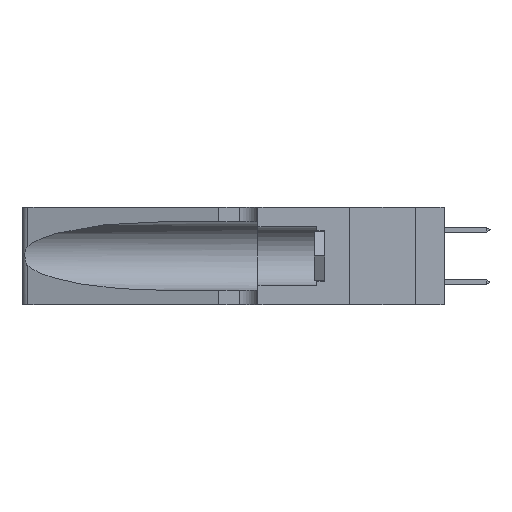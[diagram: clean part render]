
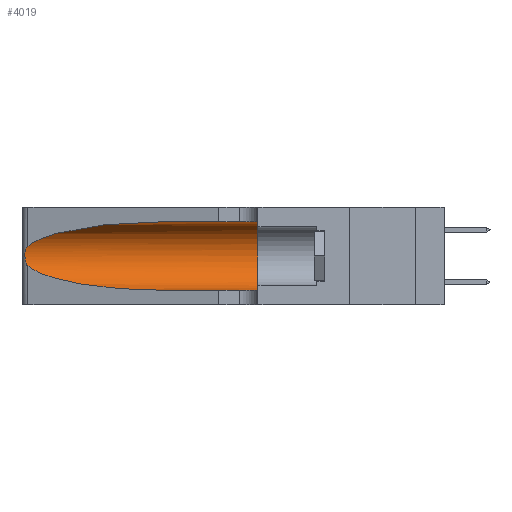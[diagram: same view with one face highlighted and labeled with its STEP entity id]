
A CAD part, left-side view. The second image highlights one B-rep face of the part: STEP entity #4019.
In plain terms, the highlighted cylindrical face has radius 3.308 mm (diameter 6.617 mm), a partial arc.
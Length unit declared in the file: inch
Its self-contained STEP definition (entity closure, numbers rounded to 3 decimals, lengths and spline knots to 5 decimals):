
#219 = CYLINDRICAL_SURFACE ( 'NONE', #3198, 0.13025 ) ;
#246 =( BOUNDED_CURVE ( )  B_SPLINE_CURVE ( 3, ( #7009, #28054, #13171, #34057 ),
 .UNSPECIFIED., .F., .F. ) 
 B_SPLINE_CURVE_WITH_KNOTS ( ( 4, 4 ),
 ( 3.44316, 4.71239 ),
 .UNSPECIFIED. ) 
 CURVE ( )  GEOMETRIC_REPRESENTATION_ITEM ( )  RATIONAL_B_SPLINE_CURVE ( ( 1., 0.87, 0.87, 1. ) ) 
 REPRESENTATION_ITEM ( '' )  );
#276 = CIRCLE ( 'NONE', #25383, 0.13025 ) ;
#822 = EDGE_LOOP ( 'NONE', ( #23058, #15701, #1438, #12077, #12701, #24550 ) ) ;
#1438 = ORIENTED_EDGE ( 'NONE', *, *, #38357, .T. ) ;
#1508 = EDGE_CURVE ( 'NONE', #5871, #12690, #15813, .T. ) ;
#1624 = CARTESIAN_POINT ( 'NONE',  ( 0.25487, 1.22718, 0.14631 ) ) ;
#2170 = CARTESIAN_POINT ( 'NONE',  ( 0.1305, 0.35, 0.31525 ) ) ;
#2357 = CARTESIAN_POINT ( 'NONE',  ( 0.25487, 1.22718, 0.22369 ) ) ;
#2413 = B_SPLINE_CURVE_WITH_KNOTS ( 'NONE', 3,
 ( #38286, #2547, #23443, #5519, #26438, #8510, #29458, #11531, #32445, #14548, #35421, #17577, #38415, #20570 ),
 .UNSPECIFIED., .F., .F.,
 ( 4, 2, 2, 2, 2, 2, 4 ),
 ( 0., 0.00027, 0.00053, 0.00107, 0.0016, 0.00187, 0.00214 ),
 .UNSPECIFIED. ) ;
#2547 = CARTESIAN_POINT ( 'NONE',  ( 0.25555, 1.22994, 0.2215 ) ) ;
#3198 = AXIS2_PLACEMENT_3D ( 'NONE', #16350, #31252, #37197 ) ;
#4019 = ADVANCED_FACE ( 'NONE', ( #16087 ), #219, .F. ) ;
#4147 = VECTOR ( 'NONE', #25179, 39.37008 ) ;
#5519 = CARTESIAN_POINT ( 'NONE',  ( 0.25787, 1.23484, 0.2124 ) ) ;
#5871 = VERTEX_POINT ( 'NONE', #16844 ) ;
#6707 = CARTESIAN_POINT ( 'NONE',  ( 0.1305, 0.35, 0.185 ) ) ;
#7009 = CARTESIAN_POINT ( 'NONE',  ( 0.25487, 1.22718, 0.14631 ) ) ;
#7465 = CARTESIAN_POINT ( 'NONE',  ( 0.18966, 0.96281, 0.31525 ) ) ;
#8510 = CARTESIAN_POINT ( 'NONE',  ( 0.26018, 1.23835, 0.19895 ) ) ;
#8898 = VERTEX_POINT ( 'NONE', #28723 ) ;
#9727 = DIRECTION ( 'NONE',  ( 0., 0., 1. ) ) ;
#10216 = LINE ( 'NONE', #20792, #4147 ) ;
#10495 = CARTESIAN_POINT ( 'NONE',  ( 0.2373, 1.15595, 0.28018 ) ) ;
#11112 = LINE ( 'NONE', #37226, #26092 ) ;
#11531 = CARTESIAN_POINT ( 'NONE',  ( 0.26075, 1.23896, 0.178 ) ) ;
#12077 = ORIENTED_EDGE ( 'NONE', *, *, #28470, .T. ) ;
#12690 = VERTEX_POINT ( 'NONE', #2357 ) ;
#12701 = ORIENTED_EDGE ( 'NONE', *, *, #36765, .F. ) ;
#12802 = CARTESIAN_POINT ( 'NONE',  ( 0.1305, 0.72297, 0.05475 ) ) ;
#13171 = CARTESIAN_POINT ( 'NONE',  ( 0.18966, 0.96281, 0.05475 ) ) ;
#13364 = DIRECTION ( 'NONE',  ( 0., -1., 0. ) ) ;
#13509 = CARTESIAN_POINT ( 'NONE',  ( 0.25487, 1.22718, 0.22369 ) ) ;
#14548 = CARTESIAN_POINT ( 'NONE',  ( 0.25856, 1.23593, 0.16098 ) ) ;
#15701 = ORIENTED_EDGE ( 'NONE', *, *, #35190, .T. ) ;
#15813 =( BOUNDED_CURVE ( )  B_SPLINE_CURVE ( 3, ( #22405, #7465, #10495, #13509 ),
 .UNSPECIFIED., .F., .F. ) 
 B_SPLINE_CURVE_WITH_KNOTS ( ( 4, 4 ),
 ( 1.5708, 2.84003 ),
 .UNSPECIFIED. ) 
 CURVE ( )  GEOMETRIC_REPRESENTATION_ITEM ( )  RATIONAL_B_SPLINE_CURVE ( ( 1., 0.87, 0.87, 1. ) ) 
 REPRESENTATION_ITEM ( '' )  );
#16087 = FACE_OUTER_BOUND ( 'NONE', #822, .T. ) ;
#16104 = VERTEX_POINT ( 'NONE', #12802 ) ;
#16350 = CARTESIAN_POINT ( 'NONE',  ( 0.1305, 1.61858, 0.185 ) ) ;
#16844 = CARTESIAN_POINT ( 'NONE',  ( 0.1305, 0.72297, 0.31525 ) ) ;
#17577 = CARTESIAN_POINT ( 'NONE',  ( 0.25639, 1.23186, 0.15144 ) ) ;
#20570 = CARTESIAN_POINT ( 'NONE',  ( 0.25487, 1.22718, 0.14631 ) ) ;
#20792 = CARTESIAN_POINT ( 'NONE',  ( 0.1305, 1.61858, 0.31525 ) ) ;
#22405 = CARTESIAN_POINT ( 'NONE',  ( 0.1305, 0.72297, 0.31525 ) ) ;
#22982 = VERTEX_POINT ( 'NONE', #2170 ) ;
#23058 = ORIENTED_EDGE ( 'NONE', *, *, #1508, .T. ) ;
#23443 = CARTESIAN_POINT ( 'NONE',  ( 0.25639, 1.23184, 0.21858 ) ) ;
#24550 = ORIENTED_EDGE ( 'NONE', *, *, #25796, .F. ) ;
#25179 = DIRECTION ( 'NONE',  ( 0., -1., 0. ) ) ;
#25383 = AXIS2_PLACEMENT_3D ( 'NONE', #6707, #27634, #9727 ) ;
#25796 = EDGE_CURVE ( 'NONE', #5871, #22982, #10216, .T. ) ;
#26092 = VECTOR ( 'NONE', #13364, 39.37008 ) ;
#26438 = CARTESIAN_POINT ( 'NONE',  ( 0.25854, 1.2359, 0.20912 ) ) ;
#27634 = DIRECTION ( 'NONE',  ( 0., 1., 0. ) ) ;
#28054 = CARTESIAN_POINT ( 'NONE',  ( 0.2373, 1.15595, 0.08982 ) ) ;
#28470 = EDGE_CURVE ( 'NONE', #16104, #8898, #11112, .T. ) ;
#28723 = CARTESIAN_POINT ( 'NONE',  ( 0.1305, 0.35, 0.05475 ) ) ;
#29458 = CARTESIAN_POINT ( 'NONE',  ( 0.26075, 1.23896, 0.19203 ) ) ;
#31252 = DIRECTION ( 'NONE',  ( 0., -1., 0. ) ) ;
#32445 = CARTESIAN_POINT ( 'NONE',  ( 0.26017, 1.23833, 0.17102 ) ) ;
#33989 = VERTEX_POINT ( 'NONE', #1624 ) ;
#34057 = CARTESIAN_POINT ( 'NONE',  ( 0.1305, 0.72297, 0.05475 ) ) ;
#35190 = EDGE_CURVE ( 'NONE', #12690, #33989, #2413, .T. ) ;
#35421 = CARTESIAN_POINT ( 'NONE',  ( 0.25789, 1.23486, 0.15765 ) ) ;
#36765 = EDGE_CURVE ( 'NONE', #22982, #8898, #276, .T. ) ;
#37197 = DIRECTION ( 'NONE',  ( 0., 0., -1. ) ) ;
#37226 = CARTESIAN_POINT ( 'NONE',  ( 0.1305, 1.61858, 0.05475 ) ) ;
#38286 = CARTESIAN_POINT ( 'NONE',  ( 0.25487, 1.22718, 0.22369 ) ) ;
#38357 = EDGE_CURVE ( 'NONE', #33989, #16104, #246, .T. ) ;
#38415 = CARTESIAN_POINT ( 'NONE',  ( 0.25555, 1.22993, 0.14849 ) ) ;
